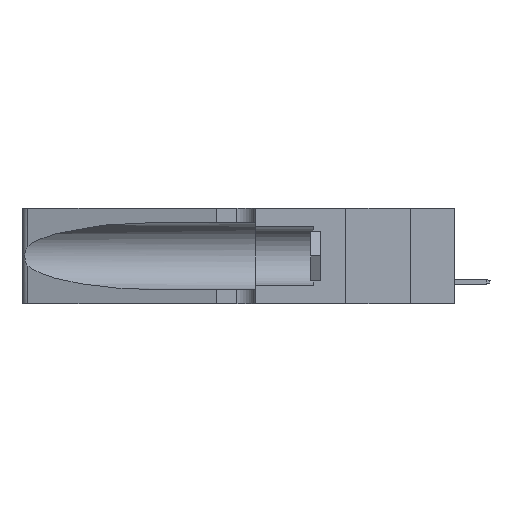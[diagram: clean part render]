
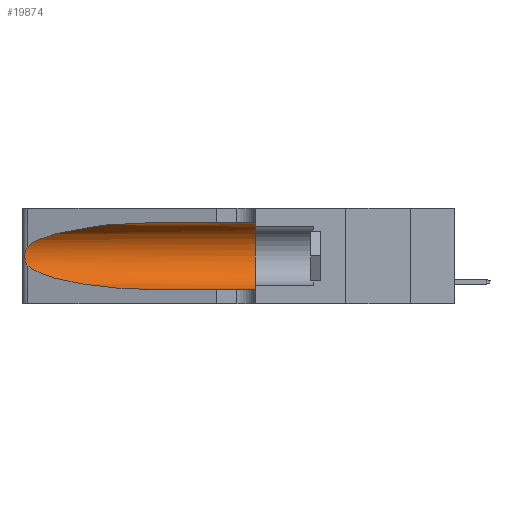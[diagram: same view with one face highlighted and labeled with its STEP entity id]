
A CAD part, left-side view. The second image highlights one B-rep face of the part: STEP entity #19874.
In plain terms, the highlighted cylindrical face has radius 3.308 mm (diameter 6.617 mm), a partial arc.
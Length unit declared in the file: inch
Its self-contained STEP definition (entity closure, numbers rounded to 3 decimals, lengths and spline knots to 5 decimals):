
#1006 = VERTEX_POINT ( 'NONE', #11882 ) ;
#1606 = CARTESIAN_POINT ( 'NONE',  ( 0.1305, 0.35, 0.185 ) ) ;
#1966 = CARTESIAN_POINT ( 'NONE',  ( 0.26075, 1.23896, 0.178 ) ) ;
#2465 = CARTESIAN_POINT ( 'NONE',  ( 0.1305, 1.61858, 0.05475 ) ) ;
#3360 = DIRECTION ( 'NONE',  ( 0., -1., 0. ) ) ;
#3769 = VERTEX_POINT ( 'NONE', #15685 ) ;
#3978 = CARTESIAN_POINT ( 'NONE',  ( 0.2373, 1.15595, 0.28018 ) ) ;
#4210 = VECTOR ( 'NONE', #19240, 39.37008 ) ;
#5517 = VERTEX_POINT ( 'NONE', #34279 ) ;
#5871 = CARTESIAN_POINT ( 'NONE',  ( 0.25487, 1.22718, 0.22369 ) ) ;
#6399 = CARTESIAN_POINT ( 'NONE',  ( 0.26018, 1.23835, 0.19895 ) ) ;
#6667 = VERTEX_POINT ( 'NONE', #21209 ) ;
#10873 = EDGE_CURVE ( 'NONE', #6667, #5517, #14865, .T. ) ;
#11482 = EDGE_LOOP ( 'NONE', ( #39086, #13615, #40900, #29067, #49438, #13116 ) ) ;
#11531 = CARTESIAN_POINT ( 'NONE',  ( 0.1305, 0.72297, 0.31525 ) ) ;
#11882 = CARTESIAN_POINT ( 'NONE',  ( 0.1305, 0.72297, 0.31525 ) ) ;
#12217 = CARTESIAN_POINT ( 'NONE',  ( 0.1305, 1.61858, 0.185 ) ) ;
#13116 = ORIENTED_EDGE ( 'NONE', *, *, #26134, .F. ) ;
#13243 = CARTESIAN_POINT ( 'NONE',  ( 0.25639, 1.23186, 0.15144 ) ) ;
#13615 = ORIENTED_EDGE ( 'NONE', *, *, #39512, .T. ) ;
#14865 =( BOUNDED_CURVE ( )  B_SPLINE_CURVE ( 3, ( #49439, #41546, #16854, #32601 ),
 .UNSPECIFIED., .F., .F. ) 
 B_SPLINE_CURVE_WITH_KNOTS ( ( 4, 4 ),
 ( 3.44316, 4.71239 ),
 .UNSPECIFIED. ) 
 CURVE ( )  GEOMETRIC_REPRESENTATION_ITEM ( )  RATIONAL_B_SPLINE_CURVE ( ( 1., 0.87, 0.87, 1. ) ) 
 REPRESENTATION_ITEM ( '' )  );
#15685 = CARTESIAN_POINT ( 'NONE',  ( 0.25487, 1.22718, 0.22369 ) ) ;
#16854 = CARTESIAN_POINT ( 'NONE',  ( 0.18966, 0.96281, 0.05475 ) ) ;
#17952 = CARTESIAN_POINT ( 'NONE',  ( 0.25555, 1.22994, 0.2215 ) ) ;
#19240 = DIRECTION ( 'NONE',  ( 0., -1., 0. ) ) ;
#19355 = CARTESIAN_POINT ( 'NONE',  ( 0.1305, 0.35, 0.05475 ) ) ;
#19620 = CARTESIAN_POINT ( 'NONE',  ( 0.1305, 1.61858, 0.31525 ) ) ;
#19874 = ADVANCED_FACE ( 'NONE', ( #29261 ), #40104, .F. ) ;
#20737 = EDGE_CURVE ( 'NONE', #1006, #3769, #49093, .T. ) ;
#21209 = CARTESIAN_POINT ( 'NONE',  ( 0.25487, 1.22718, 0.14631 ) ) ;
#21650 = AXIS2_PLACEMENT_3D ( 'NONE', #12217, #40596, #44309 ) ;
#21888 = CARTESIAN_POINT ( 'NONE',  ( 0.25639, 1.23184, 0.21858 ) ) ;
#23454 = CARTESIAN_POINT ( 'NONE',  ( 0.1305, 0.35, 0.31525 ) ) ;
#23922 = CARTESIAN_POINT ( 'NONE',  ( 0.25487, 1.22718, 0.22369 ) ) ;
#24893 = VECTOR ( 'NONE', #3360, 39.37008 ) ;
#26134 = EDGE_CURVE ( 'NONE', #1006, #28325, #47484, .T. ) ;
#26136 = VERTEX_POINT ( 'NONE', #19355 ) ;
#28325 = VERTEX_POINT ( 'NONE', #23454 ) ;
#29067 = ORIENTED_EDGE ( 'NONE', *, *, #34890, .T. ) ;
#29254 = CARTESIAN_POINT ( 'NONE',  ( 0.25555, 1.22993, 0.14849 ) ) ;
#29261 = FACE_OUTER_BOUND ( 'NONE', #11482, .T. ) ;
#31288 = CIRCLE ( 'NONE', #37977, 0.13025 ) ;
#32601 = CARTESIAN_POINT ( 'NONE',  ( 0.1305, 0.72297, 0.05475 ) ) ;
#33434 = CARTESIAN_POINT ( 'NONE',  ( 0.26017, 1.23833, 0.17102 ) ) ;
#33960 = CARTESIAN_POINT ( 'NONE',  ( 0.25856, 1.23593, 0.16098 ) ) ;
#34203 = CARTESIAN_POINT ( 'NONE',  ( 0.25854, 1.2359, 0.20912 ) ) ;
#34279 = CARTESIAN_POINT ( 'NONE',  ( 0.1305, 0.72297, 0.05475 ) ) ;
#34890 = EDGE_CURVE ( 'NONE', #5517, #26136, #46298, .T. ) ;
#37890 = CARTESIAN_POINT ( 'NONE',  ( 0.25787, 1.23484, 0.2124 ) ) ;
#37977 = AXIS2_PLACEMENT_3D ( 'NONE', #1606, #49142, #49394 ) ;
#39086 = ORIENTED_EDGE ( 'NONE', *, *, #20737, .T. ) ;
#39512 = EDGE_CURVE ( 'NONE', #3769, #6667, #47197, .T. ) ;
#40104 = CYLINDRICAL_SURFACE ( 'NONE', #21650, 0.13025 ) ;
#40596 = DIRECTION ( 'NONE',  ( 0., -1., 0. ) ) ;
#40864 = EDGE_CURVE ( 'NONE', #28325, #26136, #31288, .T. ) ;
#40900 = ORIENTED_EDGE ( 'NONE', *, *, #10873, .T. ) ;
#41546 = CARTESIAN_POINT ( 'NONE',  ( 0.2373, 1.15595, 0.08982 ) ) ;
#44309 = DIRECTION ( 'NONE',  ( 0., 0., -1. ) ) ;
#45300 = CARTESIAN_POINT ( 'NONE',  ( 0.25487, 1.22718, 0.14631 ) ) ;
#46298 = LINE ( 'NONE', #2465, #4210 ) ;
#47197 = B_SPLINE_CURVE_WITH_KNOTS ( 'NONE', 3,
 ( #5871, #17952, #21888, #37890, #34203, #6399, #49255, #1966, #33434, #33960, #50016, #13243, #29254, #45300 ),
 .UNSPECIFIED., .F., .F.,
 ( 4, 2, 2, 2, 2, 2, 4 ),
 ( 0., 0.00027, 0.00053, 0.00107, 0.0016, 0.00187, 0.00214 ),
 .UNSPECIFIED. ) ;
#47484 = LINE ( 'NONE', #19620, #24893 ) ;
#49093 =( BOUNDED_CURVE ( )  B_SPLINE_CURVE ( 3, ( #11531, #51507, #3978, #23922 ),
 .UNSPECIFIED., .F., .T. ) 
 B_SPLINE_CURVE_WITH_KNOTS ( ( 4, 4 ),
 ( 1.5708, 2.84003 ),
 .UNSPECIFIED. ) 
 CURVE ( )  GEOMETRIC_REPRESENTATION_ITEM ( )  RATIONAL_B_SPLINE_CURVE ( ( 1., 0.87, 0.87, 1. ) ) 
 REPRESENTATION_ITEM ( '' )  );
#49142 = DIRECTION ( 'NONE',  ( 0., 1., 0. ) ) ;
#49255 = CARTESIAN_POINT ( 'NONE',  ( 0.26075, 1.23896, 0.19203 ) ) ;
#49394 = DIRECTION ( 'NONE',  ( 0., 0., 1. ) ) ;
#49438 = ORIENTED_EDGE ( 'NONE', *, *, #40864, .F. ) ;
#49439 = CARTESIAN_POINT ( 'NONE',  ( 0.25487, 1.22718, 0.14631 ) ) ;
#50016 = CARTESIAN_POINT ( 'NONE',  ( 0.25789, 1.23486, 0.15765 ) ) ;
#51507 = CARTESIAN_POINT ( 'NONE',  ( 0.18966, 0.96281, 0.31525 ) ) ;
